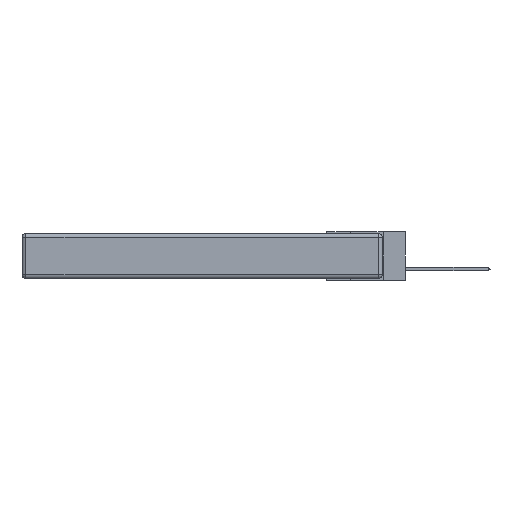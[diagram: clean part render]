
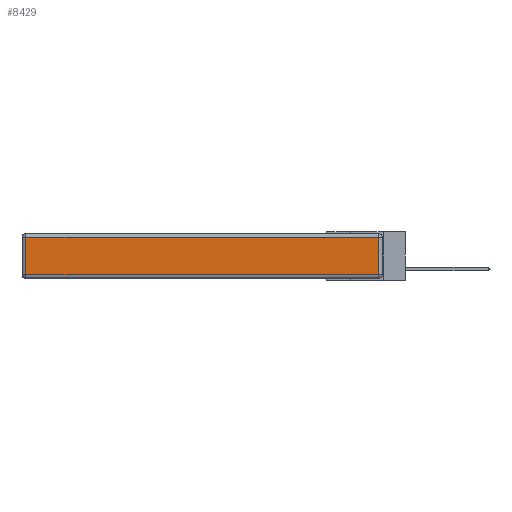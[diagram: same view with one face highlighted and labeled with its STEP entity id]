
A CAD part, left-side view. The second image highlights one B-rep face of the part: STEP entity #8429.
In plain terms, the highlighted planar face has unit normal (-1, 0, 0).
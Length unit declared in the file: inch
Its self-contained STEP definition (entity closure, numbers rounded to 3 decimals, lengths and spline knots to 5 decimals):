
#2 = EDGE_CURVE ( 'NONE', #19481, #12792, #5338, .T. ) ;
#445 = DIRECTION ( 'NONE',  ( -1., 0., 0. ) ) ;
#1839 = VERTEX_POINT ( 'NONE', #12229 ) ;
#2285 = ORIENTED_EDGE ( 'NONE', *, *, #20232, .T. ) ;
#2551 = DIRECTION ( 'NONE',  ( 0., 0., -1. ) ) ;
#2738 = CARTESIAN_POINT ( 'NONE',  ( 0., 2.75, -0.03 ) ) ;
#2740 = CARTESIAN_POINT ( 'NONE',  ( 0., 0.03, -0.343 ) ) ;
#5338 = LINE ( 'NONE', #2738, #28641 ) ;
#7111 = CARTESIAN_POINT ( 'NONE',  ( 0., 2.72, -0.03 ) ) ;
#7227 = CARTESIAN_POINT ( 'NONE',  ( 0., 0., -0.313 ) ) ;
#7370 = VECTOR ( 'NONE', #27883, 39.37008 ) ;
#7687 = EDGE_LOOP ( 'NONE', ( #2285, #18279, #24794, #23716 ) ) ;
#8429 = ADVANCED_FACE ( 'NONE', ( #15755 ), #18244, .T. ) ;
#8565 = CARTESIAN_POINT ( 'NONE',  ( 0., 2.72, -0.313 ) ) ;
#9277 = LINE ( 'NONE', #7227, #16297 ) ;
#12229 = CARTESIAN_POINT ( 'NONE',  ( 0., 0.03, -0.313 ) ) ;
#12792 = VERTEX_POINT ( 'NONE', #7111 ) ;
#13341 = CARTESIAN_POINT ( 'NONE',  ( 0., 2.72, -0.343 ) ) ;
#13814 = EDGE_CURVE ( 'NONE', #1839, #19481, #24698, .T. ) ;
#15755 = FACE_OUTER_BOUND ( 'NONE', #7687, .T. ) ;
#16139 = DIRECTION ( 'NONE',  ( 0., 0., 1. ) ) ;
#16297 = VECTOR ( 'NONE', #18851, 39.37008 ) ;
#18244 = PLANE ( 'NONE',  #24673 ) ;
#18279 = ORIENTED_EDGE ( 'NONE', *, *, #13814, .T. ) ;
#18581 = DIRECTION ( 'NONE',  ( 0., 1., 0. ) ) ;
#18851 = DIRECTION ( 'NONE',  ( 0., -1., 0. ) ) ;
#19481 = VERTEX_POINT ( 'NONE', #21698 ) ;
#20232 = EDGE_CURVE ( 'NONE', #27237, #1839, #9277, .T. ) ;
#20722 = CARTESIAN_POINT ( 'NONE',  ( 0., 0., -0.343 ) ) ;
#21078 = VECTOR ( 'NONE', #2551, 39.37008 ) ;
#21698 = CARTESIAN_POINT ( 'NONE',  ( 0., 0.03, -0.03 ) ) ;
#23716 = ORIENTED_EDGE ( 'NONE', *, *, #24864, .T. ) ;
#24673 = AXIS2_PLACEMENT_3D ( 'NONE', #20722, #445, #16139 ) ;
#24698 = LINE ( 'NONE', #2740, #7370 ) ;
#24794 = ORIENTED_EDGE ( 'NONE', *, *, #2, .T. ) ;
#24864 = EDGE_CURVE ( 'NONE', #12792, #27237, #24980, .T. ) ;
#24980 = LINE ( 'NONE', #13341, #21078 ) ;
#27237 = VERTEX_POINT ( 'NONE', #8565 ) ;
#27883 = DIRECTION ( 'NONE',  ( 0., 0., 1. ) ) ;
#28641 = VECTOR ( 'NONE', #18581, 39.37008 ) ;
